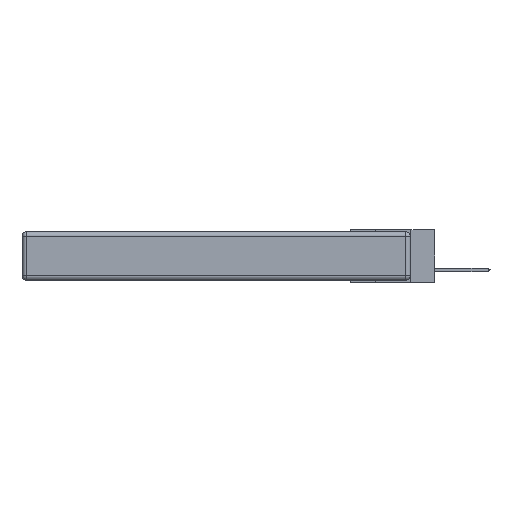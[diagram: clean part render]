
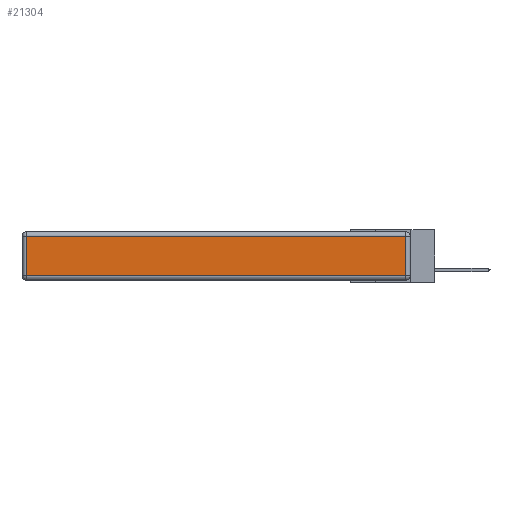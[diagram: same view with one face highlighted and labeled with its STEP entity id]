
A CAD part, left-side view. The second image highlights one B-rep face of the part: STEP entity #21304.
In plain terms, the highlighted planar face has unit normal (-1, 0, 0).
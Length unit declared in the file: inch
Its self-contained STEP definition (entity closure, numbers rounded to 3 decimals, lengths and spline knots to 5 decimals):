
#1108 = PLANE ( 'NONE',  #1369 ) ;
#1369 = AXIS2_PLACEMENT_3D ( 'NONE', #18865, #5782, #16567 ) ;
#3901 = ORIENTED_EDGE ( 'NONE', *, *, #10056, .T. ) ;
#4678 = EDGE_LOOP ( 'NONE', ( #12108, #3901, #15415, #18537 ) ) ;
#4879 = LINE ( 'NONE', #22186, #10463 ) ;
#5760 = VERTEX_POINT ( 'NONE', #10327 ) ;
#5782 = DIRECTION ( 'NONE',  ( -1., 0., 0. ) ) ;
#6466 = LINE ( 'NONE', #13524, #21059 ) ;
#6728 = LINE ( 'NONE', #14324, #15785 ) ;
#9160 = DIRECTION ( 'NONE',  ( 0., -1., 0. ) ) ;
#9944 = LINE ( 'NONE', #18192, #18585 ) ;
#10056 = EDGE_CURVE ( 'NONE', #5760, #13357, #6466, .T. ) ;
#10131 = CARTESIAN_POINT ( 'NONE',  ( 0., 0.03, -0.03 ) ) ;
#10327 = CARTESIAN_POINT ( 'NONE',  ( 0., 0.03, -0.313 ) ) ;
#10463 = VECTOR ( 'NONE', #17463, 39.37008 ) ;
#10578 = EDGE_CURVE ( 'NONE', #18868, #5760, #9944, .T. ) ;
#10887 = VERTEX_POINT ( 'NONE', #19681 ) ;
#12108 = ORIENTED_EDGE ( 'NONE', *, *, #10578, .T. ) ;
#13357 = VERTEX_POINT ( 'NONE', #10131 ) ;
#13524 = CARTESIAN_POINT ( 'NONE',  ( 0., 0.03, -0.343 ) ) ;
#14324 = CARTESIAN_POINT ( 'NONE',  ( 0., 2.72, -0.343 ) ) ;
#14611 = DIRECTION ( 'NONE',  ( 0., 0., -1. ) ) ;
#15415 = ORIENTED_EDGE ( 'NONE', *, *, #19083, .T. ) ;
#15785 = VECTOR ( 'NONE', #14611, 39.37008 ) ;
#16567 = DIRECTION ( 'NONE',  ( 0., 0., 1. ) ) ;
#17069 = EDGE_CURVE ( 'NONE', #10887, #18868, #6728, .T. ) ;
#17352 = CARTESIAN_POINT ( 'NONE',  ( 0., 2.72, -0.313 ) ) ;
#17463 = DIRECTION ( 'NONE',  ( 0., 1., 0. ) ) ;
#18192 = CARTESIAN_POINT ( 'NONE',  ( 0., 0., -0.313 ) ) ;
#18537 = ORIENTED_EDGE ( 'NONE', *, *, #17069, .T. ) ;
#18585 = VECTOR ( 'NONE', #9160, 39.37008 ) ;
#18865 = CARTESIAN_POINT ( 'NONE',  ( 0., 0., -0.343 ) ) ;
#18868 = VERTEX_POINT ( 'NONE', #17352 ) ;
#19083 = EDGE_CURVE ( 'NONE', #13357, #10887, #4879, .T. ) ;
#19681 = CARTESIAN_POINT ( 'NONE',  ( 0., 2.72, -0.03 ) ) ;
#21059 = VECTOR ( 'NONE', #24435, 39.37008 ) ;
#21304 = ADVANCED_FACE ( 'NONE', ( #23415 ), #1108, .T. ) ;
#22186 = CARTESIAN_POINT ( 'NONE',  ( 0., 2.75, -0.03 ) ) ;
#23415 = FACE_OUTER_BOUND ( 'NONE', #4678, .T. ) ;
#24435 = DIRECTION ( 'NONE',  ( 0., 0., 1. ) ) ;
